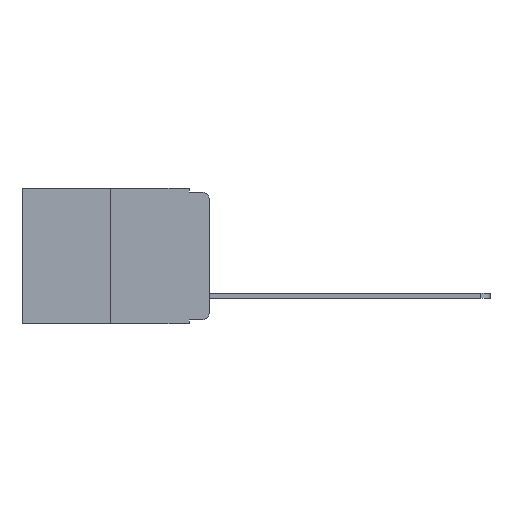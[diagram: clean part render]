
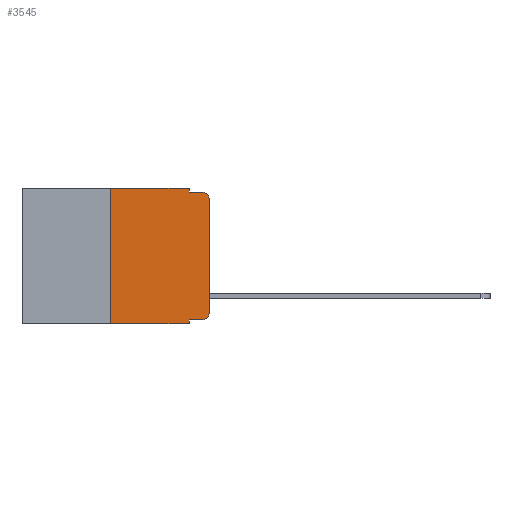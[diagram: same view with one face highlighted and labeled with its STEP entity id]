
A CAD part, left-side view. The second image highlights one B-rep face of the part: STEP entity #3545.
In plain terms, the highlighted planar face has unit normal (-1, 0, 0).
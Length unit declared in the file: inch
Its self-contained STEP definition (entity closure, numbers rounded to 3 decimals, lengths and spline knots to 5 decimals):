
#109 = VERTEX_POINT ( 'NONE', #6316 ) ;
#320 = VECTOR ( 'NONE', #7844, 39.37008 ) ;
#526 = DIRECTION ( 'NONE',  ( 0., -1., 0. ) ) ;
#688 = LINE ( 'NONE', #2787, #5006 ) ;
#832 = VERTEX_POINT ( 'NONE', #6751 ) ;
#1045 = DIRECTION ( 'NONE',  ( -1., 0., 0. ) ) ;
#1178 = DIRECTION ( 'NONE',  ( 1., 0., 0. ) ) ;
#1224 = VERTEX_POINT ( 'NONE', #6769 ) ;
#1310 = VERTEX_POINT ( 'NONE', #7337 ) ;
#1331 = DIRECTION ( 'NONE',  ( 0., 0., -1. ) ) ;
#1574 = VERTEX_POINT ( 'NONE', #8344 ) ;
#1702 = EDGE_CURVE ( 'NONE', #8343, #832, #8412, .T. ) ;
#1886 = CARTESIAN_POINT ( 'NONE',  ( 0., 0.25, 0. ) ) ;
#1922 = VERTEX_POINT ( 'NONE', #7280 ) ;
#1925 = DIRECTION ( 'NONE',  ( 0., 0., 1. ) ) ;
#1996 = CARTESIAN_POINT ( 'NONE',  ( 0., 0.473, 0. ) ) ;
#2438 = VERTEX_POINT ( 'NONE', #3613 ) ;
#2596 = CIRCLE ( 'NONE', #6580, 0.02 ) ;
#2787 = CARTESIAN_POINT ( 'NONE',  ( 0., 0.25, 0. ) ) ;
#2853 = VECTOR ( 'NONE', #6711, 39.37008 ) ;
#3101 = VECTOR ( 'NONE', #3527, 39.37008 ) ;
#3312 = PLANE ( 'NONE',  #3950 ) ;
#3347 = LINE ( 'NONE', #5417, #3101 ) ;
#3527 = DIRECTION ( 'NONE',  ( 0., 0., 1. ) ) ;
#3545 = ADVANCED_FACE ( 'NONE', ( #8544 ), #3312, .F. ) ;
#3574 = CARTESIAN_POINT ( 'NONE',  ( 0., 0.02, -0.03 ) ) ;
#3613 = CARTESIAN_POINT ( 'NONE',  ( 0., 0.02, -0.01 ) ) ;
#3703 = VERTEX_POINT ( 'NONE', #8518 ) ;
#3950 = AXIS2_PLACEMENT_3D ( 'NONE', #1996, #1178, #1331 ) ;
#4571 = DIRECTION ( 'NONE',  ( 0., 0., -1. ) ) ;
#4617 = DIRECTION ( 'NONE',  ( 0., 0., -1. ) ) ;
#5006 = VECTOR ( 'NONE', #1925, 39.37008 ) ;
#5417 = CARTESIAN_POINT ( 'NONE',  ( 0., 0., 0. ) ) ;
#5442 = ORIENTED_EDGE ( 'NONE', *, *, #7924, .T. ) ;
#5444 = ORIENTED_EDGE ( 'NONE', *, *, #1702, .F. ) ;
#5456 = ORIENTED_EDGE ( 'NONE', *, *, #8482, .F. ) ;
#5472 = ORIENTED_EDGE ( 'NONE', *, *, #8483, .F. ) ;
#5484 = ORIENTED_EDGE ( 'NONE', *, *, #8284, .T. ) ;
#5505 = CIRCLE ( 'NONE', #6593, 0.02 ) ;
#5541 = ORIENTED_EDGE ( 'NONE', *, *, #8316, .T. ) ;
#5600 = ORIENTED_EDGE ( 'NONE', *, *, #8594, .T. ) ;
#5612 = ORIENTED_EDGE ( 'NONE', *, *, #8495, .F. ) ;
#5639 = ORIENTED_EDGE ( 'NONE', *, *, #8515, .F. ) ;
#5647 = ORIENTED_EDGE ( 'NONE', *, *, #8592, .T. ) ;
#5764 = EDGE_LOOP ( 'NONE', ( #5484, #5541, #5456, #5472, #5444, #5612, #5442, #5639, #5647, #5600 ) ) ;
#5813 = CARTESIAN_POINT ( 'NONE',  ( 0., 0.473, -0.343 ) ) ;
#6124 = CARTESIAN_POINT ( 'NONE',  ( 0., 0.02, -0.313 ) ) ;
#6182 = LINE ( 'NONE', #5813, #7548 ) ;
#6316 = CARTESIAN_POINT ( 'NONE',  ( 0., 0.02, -0.333 ) ) ;
#6580 = AXIS2_PLACEMENT_3D ( 'NONE', #6124, #1045, #6757 ) ;
#6593 = AXIS2_PLACEMENT_3D ( 'NONE', #3574, #8388, #4571 ) ;
#6711 = DIRECTION ( 'NONE',  ( 0., -1., 0. ) ) ;
#6751 = CARTESIAN_POINT ( 'NONE',  ( 0., 0.051, 0. ) ) ;
#6757 = DIRECTION ( 'NONE',  ( 0., 0., -1. ) ) ;
#6769 = CARTESIAN_POINT ( 'NONE',  ( 0., 0., -0.313 ) ) ;
#6772 = LINE ( 'NONE', #9354, #9400 ) ;
#6954 = LINE ( 'NONE', #8409, #8270 ) ;
#7280 = CARTESIAN_POINT ( 'NONE',  ( 0., 0.051, -0.343 ) ) ;
#7303 = CARTESIAN_POINT ( 'NONE',  ( 0., 0.051, -0.333 ) ) ;
#7337 = CARTESIAN_POINT ( 'NONE',  ( 0., 0.051, -0.01 ) ) ;
#7548 = VECTOR ( 'NONE', #526, 39.37008 ) ;
#7553 = CARTESIAN_POINT ( 'NONE',  ( 0., 0., -0.03 ) ) ;
#7821 = CARTESIAN_POINT ( 'NONE',  ( 0., 0.051, -0.01 ) ) ;
#7826 = VERTEX_POINT ( 'NONE', #7553 ) ;
#7844 = DIRECTION ( 'NONE',  ( 0., -1., 0. ) ) ;
#7924 = EDGE_CURVE ( 'NONE', #1574, #1922, #6182, .T. ) ;
#8074 = LINE ( 'NONE', #7303, #320 ) ;
#8226 = VECTOR ( 'NONE', #9005, 39.37008 ) ;
#8270 = VECTOR ( 'NONE', #8941, 39.37008 ) ;
#8284 = EDGE_CURVE ( 'NONE', #1224, #7826, #3347, .T. ) ;
#8316 = EDGE_CURVE ( 'NONE', #7826, #2438, #5505, .T. ) ;
#8343 = VERTEX_POINT ( 'NONE', #1886 ) ;
#8344 = CARTESIAN_POINT ( 'NONE',  ( 0., 0.25, -0.343 ) ) ;
#8388 = DIRECTION ( 'NONE',  ( -1., 0., 0. ) ) ;
#8409 = CARTESIAN_POINT ( 'NONE',  ( 0., 0.051, 0. ) ) ;
#8412 = LINE ( 'NONE', #9120, #8226 ) ;
#8446 = LINE ( 'NONE', #7821, #2853 ) ;
#8482 = EDGE_CURVE ( 'NONE', #1310, #2438, #8446, .T. ) ;
#8483 = EDGE_CURVE ( 'NONE', #832, #1310, #6954, .T. ) ;
#8495 = EDGE_CURVE ( 'NONE', #1574, #8343, #688, .T. ) ;
#8515 = EDGE_CURVE ( 'NONE', #3703, #1922, #6772, .T. ) ;
#8518 = CARTESIAN_POINT ( 'NONE',  ( 0., 0.051, -0.333 ) ) ;
#8544 = FACE_OUTER_BOUND ( 'NONE', #5764, .T. ) ;
#8592 = EDGE_CURVE ( 'NONE', #3703, #109, #8074, .T. ) ;
#8594 = EDGE_CURVE ( 'NONE', #109, #1224, #2596, .T. ) ;
#8941 = DIRECTION ( 'NONE',  ( 0., 0., -1. ) ) ;
#9005 = DIRECTION ( 'NONE',  ( 0., -1., 0. ) ) ;
#9120 = CARTESIAN_POINT ( 'NONE',  ( 0., 0.473, 0. ) ) ;
#9354 = CARTESIAN_POINT ( 'NONE',  ( 0., 0.051, 0. ) ) ;
#9400 = VECTOR ( 'NONE', #4617, 39.37008 ) ;
